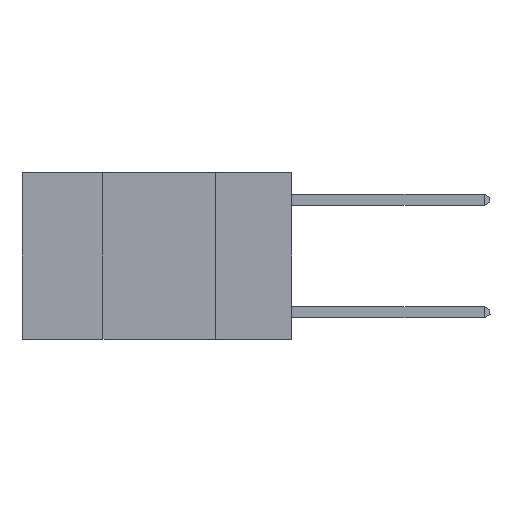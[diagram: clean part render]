
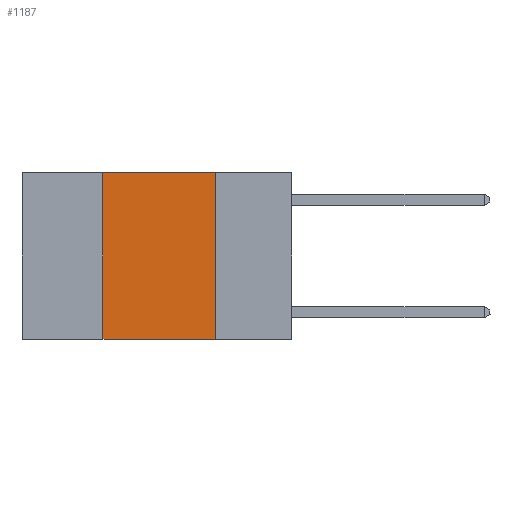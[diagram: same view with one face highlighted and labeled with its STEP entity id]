
A CAD part, left-side view. The second image highlights one B-rep face of the part: STEP entity #1187.
In plain terms, the highlighted planar face has unit normal (-1, 0, 0).
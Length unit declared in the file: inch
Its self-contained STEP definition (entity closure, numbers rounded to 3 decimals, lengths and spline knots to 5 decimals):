
#266 = CARTESIAN_POINT ( 'NONE',  ( 0., 0.17, 0. ) ) ;
#524 = EDGE_CURVE ( 'NONE', #3479, #6732, #4627, .T. ) ;
#999 = EDGE_CURVE ( 'NONE', #11004, #3479, #5571, .T. ) ;
#1077 = CARTESIAN_POINT ( 'NONE',  ( 0., 0.17, -0.37 ) ) ;
#1130 = EDGE_CURVE ( 'NONE', #11004, #5441, #6707, .T. ) ;
#1187 = ADVANCED_FACE ( 'NONE', ( #2958 ), #8123, .F. ) ;
#1422 = ORIENTED_EDGE ( 'NONE', *, *, #1130, .T. ) ;
#1942 = DIRECTION ( 'NONE',  ( 0., 0., -1. ) ) ;
#2178 = VECTOR ( 'NONE', #8811, 39.37008 ) ;
#2958 = FACE_OUTER_BOUND ( 'NONE', #3052, .T. ) ;
#3052 = EDGE_LOOP ( 'NONE', ( #3201, #8070, #3209, #1422 ) ) ;
#3201 = ORIENTED_EDGE ( 'NONE', *, *, #11932, .F. ) ;
#3209 = ORIENTED_EDGE ( 'NONE', *, *, #999, .F. ) ;
#3479 = VERTEX_POINT ( 'NONE', #5287 ) ;
#4627 = LINE ( 'NONE', #9631, #2178 ) ;
#5287 = CARTESIAN_POINT ( 'NONE',  ( 0., 0.42, 0. ) ) ;
#5441 = VERTEX_POINT ( 'NONE', #1077 ) ;
#5571 = LINE ( 'NONE', #11261, #10485 ) ;
#6707 = LINE ( 'NONE', #10104, #9303 ) ;
#6732 = VERTEX_POINT ( 'NONE', #11889 ) ;
#7605 = AXIS2_PLACEMENT_3D ( 'NONE', #12854, #8875, #1942 ) ;
#8070 = ORIENTED_EDGE ( 'NONE', *, *, #524, .F. ) ;
#8123 = PLANE ( 'NONE',  #7605 ) ;
#8454 = DIRECTION ( 'NONE',  ( 0., 0., 1. ) ) ;
#8811 = DIRECTION ( 'NONE',  ( 0., -1., 0. ) ) ;
#8875 = DIRECTION ( 'NONE',  ( 1., 0., 0. ) ) ;
#9303 = VECTOR ( 'NONE', #9620, 39.37008 ) ;
#9620 = DIRECTION ( 'NONE',  ( 0., -1., 0. ) ) ;
#9631 = CARTESIAN_POINT ( 'NONE',  ( 0., 0.6, 0. ) ) ;
#10104 = CARTESIAN_POINT ( 'NONE',  ( 0., 0.6, -0.37 ) ) ;
#10225 = LINE ( 'NONE', #266, #12679 ) ;
#10485 = VECTOR ( 'NONE', #8454, 39.37008 ) ;
#11004 = VERTEX_POINT ( 'NONE', #11084 ) ;
#11084 = CARTESIAN_POINT ( 'NONE',  ( 0., 0.42, -0.37 ) ) ;
#11261 = CARTESIAN_POINT ( 'NONE',  ( 0., 0.42, 0. ) ) ;
#11397 = DIRECTION ( 'NONE',  ( 0., 0., -1. ) ) ;
#11889 = CARTESIAN_POINT ( 'NONE',  ( 0., 0.17, 0. ) ) ;
#11932 = EDGE_CURVE ( 'NONE', #6732, #5441, #10225, .T. ) ;
#12679 = VECTOR ( 'NONE', #11397, 39.37008 ) ;
#12854 = CARTESIAN_POINT ( 'NONE',  ( 0., 0.6, 0. ) ) ;
